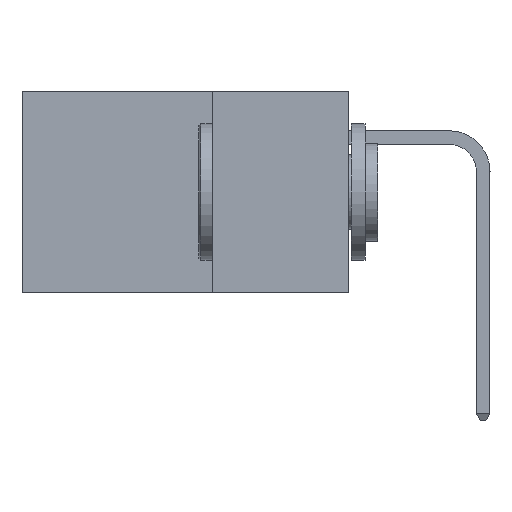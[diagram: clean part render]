
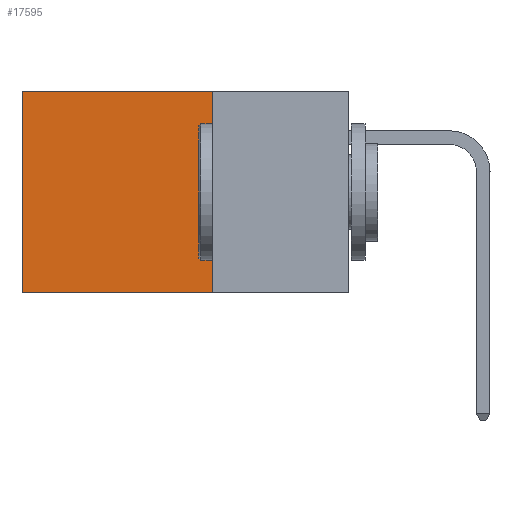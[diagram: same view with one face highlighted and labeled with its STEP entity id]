
A CAD part, left-side view. The second image highlights one B-rep face of the part: STEP entity #17595.
In plain terms, the highlighted planar face has unit normal (-1, 0, 0).
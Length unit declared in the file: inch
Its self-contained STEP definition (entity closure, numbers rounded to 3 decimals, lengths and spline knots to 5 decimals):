
#3102 = VECTOR ( 'NONE', #17435, 39.37008 ) ;
#3382 = CARTESIAN_POINT ( 'NONE',  ( 0.2875, 0.25, 0. ) ) ;
#5121 = DIRECTION ( 'NONE',  ( 0., 1., 0. ) ) ;
#5865 = EDGE_LOOP ( 'NONE', ( #35514, #29938, #9960, #12640 ) ) ;
#6633 = LINE ( 'NONE', #7063, #34372 ) ;
#7063 = CARTESIAN_POINT ( 'NONE',  ( 0.2875, 0.25, -0.37 ) ) ;
#8837 = CARTESIAN_POINT ( 'NONE',  ( 0.2875, 0.25, 0. ) ) ;
#9488 = DIRECTION ( 'NONE',  ( 0., 0., -1. ) ) ;
#9960 = ORIENTED_EDGE ( 'NONE', *, *, #35880, .F. ) ;
#10737 = EDGE_CURVE ( 'NONE', #14652, #14387, #29756, .T. ) ;
#12640 = ORIENTED_EDGE ( 'NONE', *, *, #10737, .T. ) ;
#13588 = VECTOR ( 'NONE', #33701, 39.37008 ) ;
#13677 = VECTOR ( 'NONE', #5121, 39.37008 ) ;
#14387 = VERTEX_POINT ( 'NONE', #16623 ) ;
#14647 = VERTEX_POINT ( 'NONE', #32073 ) ;
#14652 = VERTEX_POINT ( 'NONE', #3382 ) ;
#16333 = AXIS2_PLACEMENT_3D ( 'NONE', #35001, #26558, #9488 ) ;
#16623 = CARTESIAN_POINT ( 'NONE',  ( 0.2875, 0.6, 0. ) ) ;
#17291 = EDGE_CURVE ( 'NONE', #14387, #32285, #21179, .T. ) ;
#17435 = DIRECTION ( 'NONE',  ( 0., 0., -1. ) ) ;
#17595 = ADVANCED_FACE ( 'NONE', ( #18029 ), #23700, .F. ) ;
#18029 = FACE_OUTER_BOUND ( 'NONE', #5865, .T. ) ;
#18428 = LINE ( 'NONE', #8837, #3102 ) ;
#19432 = EDGE_CURVE ( 'NONE', #14647, #32285, #6633, .T. ) ;
#21179 = LINE ( 'NONE', #27957, #13588 ) ;
#22296 = CARTESIAN_POINT ( 'NONE',  ( 0.2875, 0.25, 0. ) ) ;
#23700 = PLANE ( 'NONE',  #16333 ) ;
#26558 = DIRECTION ( 'NONE',  ( 1., 0., 0. ) ) ;
#27957 = CARTESIAN_POINT ( 'NONE',  ( 0.2875, 0.6, 0. ) ) ;
#29756 = LINE ( 'NONE', #22296, #13677 ) ;
#29938 = ORIENTED_EDGE ( 'NONE', *, *, #19432, .F. ) ;
#29956 = DIRECTION ( 'NONE',  ( 0., 1., 0. ) ) ;
#32073 = CARTESIAN_POINT ( 'NONE',  ( 0.2875, 0.25, -0.37 ) ) ;
#32285 = VERTEX_POINT ( 'NONE', #34449 ) ;
#33701 = DIRECTION ( 'NONE',  ( 0., 0., -1. ) ) ;
#34372 = VECTOR ( 'NONE', #29956, 39.37008 ) ;
#34449 = CARTESIAN_POINT ( 'NONE',  ( 0.2875, 0.6, -0.37 ) ) ;
#35001 = CARTESIAN_POINT ( 'NONE',  ( 0.2875, 0.25, 0. ) ) ;
#35514 = ORIENTED_EDGE ( 'NONE', *, *, #17291, .T. ) ;
#35880 = EDGE_CURVE ( 'NONE', #14652, #14647, #18428, .T. ) ;
